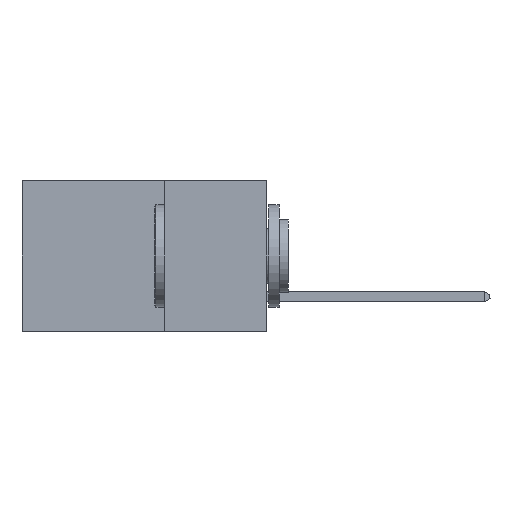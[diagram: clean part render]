
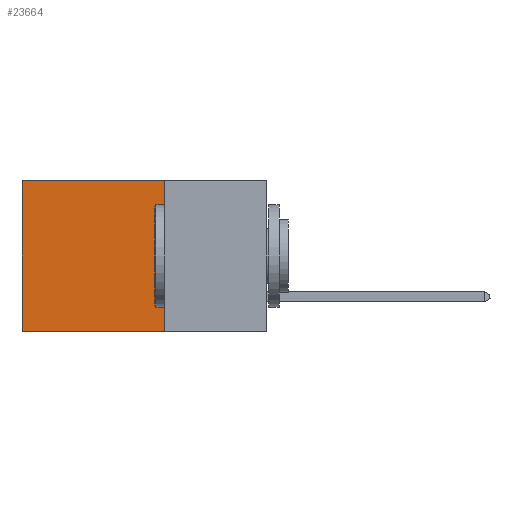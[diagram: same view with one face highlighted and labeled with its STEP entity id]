
A CAD part, left-side view. The second image highlights one B-rep face of the part: STEP entity #23664.
In plain terms, the highlighted planar face has unit normal (-1, 0, 0).
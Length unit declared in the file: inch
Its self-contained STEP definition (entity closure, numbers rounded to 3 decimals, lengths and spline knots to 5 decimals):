
#2762 = VERTEX_POINT ( 'NONE', #19127 ) ;
#3496 = DIRECTION ( 'NONE',  ( 0., 0., -1. ) ) ;
#3503 = EDGE_CURVE ( 'NONE', #2762, #23764, #12512, .T. ) ;
#4301 = CARTESIAN_POINT ( 'NONE',  ( 0.2875, 0.25, 0. ) ) ;
#5902 = ORIENTED_EDGE ( 'NONE', *, *, #8613, .F. ) ;
#5985 = CARTESIAN_POINT ( 'NONE',  ( 0.2875, 0.25, 0. ) ) ;
#7255 = VECTOR ( 'NONE', #17664, 39.37008 ) ;
#8602 = DIRECTION ( 'NONE',  ( 1., 0., 0. ) ) ;
#8613 = EDGE_CURVE ( 'NONE', #32617, #2762, #21968, .T. ) ;
#9164 = CARTESIAN_POINT ( 'NONE',  ( 0.2875, 0.6, -0.37 ) ) ;
#9813 = ORIENTED_EDGE ( 'NONE', *, *, #3503, .F. ) ;
#11101 = LINE ( 'NONE', #4301, #24799 ) ;
#11888 = DIRECTION ( 'NONE',  ( 0., 0., -1. ) ) ;
#12430 = DIRECTION ( 'NONE',  ( 0., 1., 0. ) ) ;
#12504 = CARTESIAN_POINT ( 'NONE',  ( 0.2875, 0.25, -0.37 ) ) ;
#12512 = LINE ( 'NONE', #12504, #7255 ) ;
#15171 = ORIENTED_EDGE ( 'NONE', *, *, #17511, .T. ) ;
#17511 = EDGE_CURVE ( 'NONE', #32617, #24251, #11101, .T. ) ;
#17664 = DIRECTION ( 'NONE',  ( 0., 1., 0. ) ) ;
#18990 = VECTOR ( 'NONE', #26418, 39.37008 ) ;
#19127 = CARTESIAN_POINT ( 'NONE',  ( 0.2875, 0.25, -0.37 ) ) ;
#21220 = ORIENTED_EDGE ( 'NONE', *, *, #21857, .T. ) ;
#21307 = PLANE ( 'NONE',  #22582 ) ;
#21857 = EDGE_CURVE ( 'NONE', #24251, #23764, #29119, .T. ) ;
#21968 = LINE ( 'NONE', #33406, #23163 ) ;
#22582 = AXIS2_PLACEMENT_3D ( 'NONE', #5985, #8602, #3496 ) ;
#23163 = VECTOR ( 'NONE', #11888, 39.37008 ) ;
#23664 = ADVANCED_FACE ( 'NONE', ( #30591 ), #21307, .F. ) ;
#23692 = EDGE_LOOP ( 'NONE', ( #21220, #9813, #5902, #15171 ) ) ;
#23764 = VERTEX_POINT ( 'NONE', #9164 ) ;
#24251 = VERTEX_POINT ( 'NONE', #27472 ) ;
#24799 = VECTOR ( 'NONE', #12430, 39.37008 ) ;
#26418 = DIRECTION ( 'NONE',  ( 0., 0., -1. ) ) ;
#27250 = CARTESIAN_POINT ( 'NONE',  ( 0.2875, 0.25, 0. ) ) ;
#27472 = CARTESIAN_POINT ( 'NONE',  ( 0.2875, 0.6, 0. ) ) ;
#28805 = CARTESIAN_POINT ( 'NONE',  ( 0.2875, 0.6, 0. ) ) ;
#29119 = LINE ( 'NONE', #28805, #18990 ) ;
#30591 = FACE_OUTER_BOUND ( 'NONE', #23692, .T. ) ;
#32617 = VERTEX_POINT ( 'NONE', #27250 ) ;
#33406 = CARTESIAN_POINT ( 'NONE',  ( 0.2875, 0.25, 0. ) ) ;
